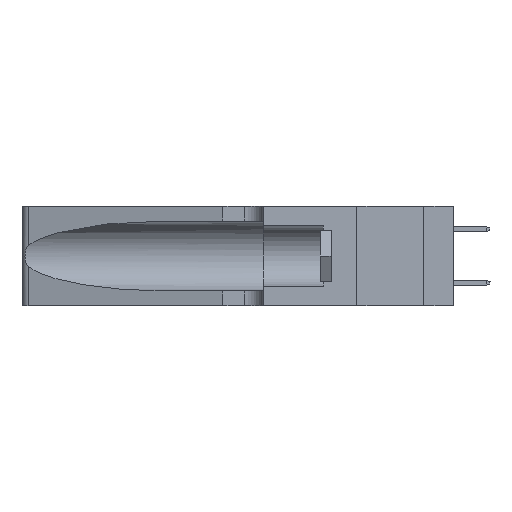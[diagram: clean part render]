
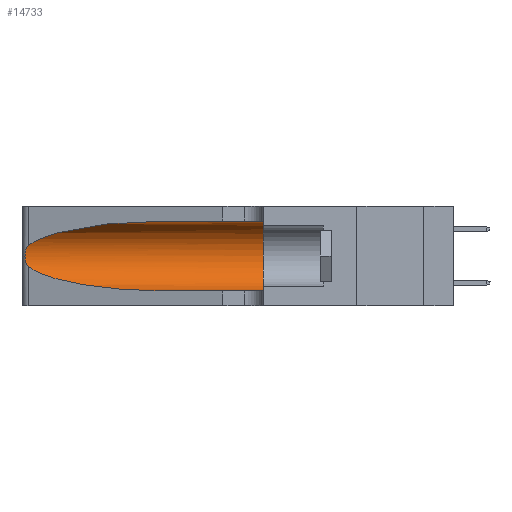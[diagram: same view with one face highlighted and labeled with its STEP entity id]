
A CAD part, left-side view. The second image highlights one B-rep face of the part: STEP entity #14733.
In plain terms, the highlighted cylindrical face has radius 3.308 mm (diameter 6.617 mm), a partial arc.
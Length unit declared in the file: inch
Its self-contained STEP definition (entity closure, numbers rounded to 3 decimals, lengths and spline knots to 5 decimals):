
#39 = CYLINDRICAL_SURFACE ( 'NONE', #864, 0.13025 ) ;
#864 = AXIS2_PLACEMENT_3D ( 'NONE', #15538, #2279, #7613 ) ;
#965 = ORIENTED_EDGE ( 'NONE', *, *, #1221, .F. ) ;
#1221 = EDGE_CURVE ( 'NONE', #31460, #3179, #30918, .T. ) ;
#1354 = CARTESIAN_POINT ( 'NONE',  ( 0.26075, 1.23896, 0.178 ) ) ;
#1527 = CARTESIAN_POINT ( 'NONE',  ( 0.26075, 1.23896, 0.19203 ) ) ;
#1654 = VERTEX_POINT ( 'NONE', #29854 ) ;
#1862 = VERTEX_POINT ( 'NONE', #2732 ) ;
#2131 = EDGE_CURVE ( 'NONE', #1654, #1862, #22072, .T. ) ;
#2279 = DIRECTION ( 'NONE',  ( 0., -1., 0. ) ) ;
#2346 = ORIENTED_EDGE ( 'NONE', *, *, #2131, .T. ) ;
#2530 = CARTESIAN_POINT ( 'NONE',  ( 0.1305, 0.72297, 0.31525 ) ) ;
#2732 = CARTESIAN_POINT ( 'NONE',  ( 0.25487, 1.22718, 0.14631 ) ) ;
#3179 = VERTEX_POINT ( 'NONE', #7120 ) ;
#5054 = CARTESIAN_POINT ( 'NONE',  ( 0.1305, 0.72297, 0.05475 ) ) ;
#5579 = AXIS2_PLACEMENT_3D ( 'NONE', #21646, #8551, #21817 ) ;
#6100 = ORIENTED_EDGE ( 'NONE', *, *, #20567, .F. ) ;
#6348 = CARTESIAN_POINT ( 'NONE',  ( 0.25487, 1.22718, 0.22369 ) ) ;
#6790 = LINE ( 'NONE', #27851, #25215 ) ;
#7036 = CARTESIAN_POINT ( 'NONE',  ( 0.25487, 1.22718, 0.14631 ) ) ;
#7120 = CARTESIAN_POINT ( 'NONE',  ( 0.1305, 0.35, 0.05475 ) ) ;
#7125 = CARTESIAN_POINT ( 'NONE',  ( 0.25487, 1.22718, 0.14631 ) ) ;
#7238 = CARTESIAN_POINT ( 'NONE',  ( 0.1305, 1.61858, 0.05475 ) ) ;
#7613 = DIRECTION ( 'NONE',  ( 0., 0., -1. ) ) ;
#8551 = DIRECTION ( 'NONE',  ( 0., 1., 0. ) ) ;
#9964 = CARTESIAN_POINT ( 'NONE',  ( 0.18966, 0.96281, 0.31525 ) ) ;
#10334 = LINE ( 'NONE', #7238, #25670 ) ;
#11707 = CARTESIAN_POINT ( 'NONE',  ( 0.25639, 1.23186, 0.15144 ) ) ;
#12054 = CARTESIAN_POINT ( 'NONE',  ( 0.25555, 1.22993, 0.14849 ) ) ;
#13056 = CARTESIAN_POINT ( 'NONE',  ( 0.25487, 1.22718, 0.22369 ) ) ;
#13820 = ORIENTED_EDGE ( 'NONE', *, *, #17818, .T. ) ;
#14646 = CARTESIAN_POINT ( 'NONE',  ( 0.1305, 0.35, 0.31525 ) ) ;
#14733 = ADVANCED_FACE ( 'NONE', ( #15710 ), #39, .F. ) ;
#15238 = EDGE_CURVE ( 'NONE', #31876, #3179, #10334, .T. ) ;
#15380 = CARTESIAN_POINT ( 'NONE',  ( 0.18966, 0.96281, 0.05475 ) ) ;
#15538 = CARTESIAN_POINT ( 'NONE',  ( 0.1305, 1.61858, 0.185 ) ) ;
#15710 = FACE_OUTER_BOUND ( 'NONE', #19893, .T. ) ;
#15809 = CARTESIAN_POINT ( 'NONE',  ( 0.2373, 1.15595, 0.28018 ) ) ;
#16860 = CARTESIAN_POINT ( 'NONE',  ( 0.25854, 1.2359, 0.20912 ) ) ;
#17818 = EDGE_CURVE ( 'NONE', #1862, #31876, #25485, .T. ) ;
#19546 =( BOUNDED_CURVE ( )  B_SPLINE_CURVE ( 3, ( #2530, #9964, #15809, #13056 ),
 .UNSPECIFIED., .F., .F. ) 
 B_SPLINE_CURVE_WITH_KNOTS ( ( 4, 4 ),
 ( 1.5708, 2.84003 ),
 .UNSPECIFIED. ) 
 CURVE ( )  GEOMETRIC_REPRESENTATION_ITEM ( )  RATIONAL_B_SPLINE_CURVE ( ( 1., 0.87, 0.87, 1. ) ) 
 REPRESENTATION_ITEM ( '' )  );
#19893 = EDGE_LOOP ( 'NONE', ( #32483, #2346, #13820, #28740, #965, #6100 ) ) ;
#20567 = EDGE_CURVE ( 'NONE', #24941, #31460, #6790, .T. ) ;
#21646 = CARTESIAN_POINT ( 'NONE',  ( 0.1305, 0.35, 0.185 ) ) ;
#21817 = DIRECTION ( 'NONE',  ( 0., 0., 1. ) ) ;
#22072 = B_SPLINE_CURVE_WITH_KNOTS ( 'NONE', 3,
 ( #6348, #24802, #22586, #30490, #16860, #27404, #1527, #1354, #30156, #27752, #25148, #11707, #12054, #7036 ),
 .UNSPECIFIED., .F., .F.,
 ( 4, 2, 2, 2, 2, 2, 4 ),
 ( 0., 0.00027, 0.00053, 0.00107, 0.0016, 0.00187, 0.00214 ),
 .UNSPECIFIED. ) ;
#22586 = CARTESIAN_POINT ( 'NONE',  ( 0.25639, 1.23184, 0.21858 ) ) ;
#22842 = CARTESIAN_POINT ( 'NONE',  ( 0.2373, 1.15595, 0.08982 ) ) ;
#23287 = DIRECTION ( 'NONE',  ( 0., -1., 0. ) ) ;
#24802 = CARTESIAN_POINT ( 'NONE',  ( 0.25555, 1.22994, 0.2215 ) ) ;
#24941 = VERTEX_POINT ( 'NONE', #30001 ) ;
#25148 = CARTESIAN_POINT ( 'NONE',  ( 0.25789, 1.23486, 0.15765 ) ) ;
#25215 = VECTOR ( 'NONE', #30588, 39.37008 ) ;
#25485 =( BOUNDED_CURVE ( )  B_SPLINE_CURVE ( 3, ( #7125, #22842, #15380, #5054 ),
 .UNSPECIFIED., .F., .F. ) 
 B_SPLINE_CURVE_WITH_KNOTS ( ( 4, 4 ),
 ( 3.44316, 4.71239 ),
 .UNSPECIFIED. ) 
 CURVE ( )  GEOMETRIC_REPRESENTATION_ITEM ( )  RATIONAL_B_SPLINE_CURVE ( ( 1., 0.87, 0.87, 1. ) ) 
 REPRESENTATION_ITEM ( '' )  );
#25670 = VECTOR ( 'NONE', #23287, 39.37008 ) ;
#27266 = EDGE_CURVE ( 'NONE', #24941, #1654, #19546, .T. ) ;
#27404 = CARTESIAN_POINT ( 'NONE',  ( 0.26018, 1.23835, 0.19895 ) ) ;
#27752 = CARTESIAN_POINT ( 'NONE',  ( 0.25856, 1.23593, 0.16098 ) ) ;
#27851 = CARTESIAN_POINT ( 'NONE',  ( 0.1305, 1.61858, 0.31525 ) ) ;
#28740 = ORIENTED_EDGE ( 'NONE', *, *, #15238, .T. ) ;
#29854 = CARTESIAN_POINT ( 'NONE',  ( 0.25487, 1.22718, 0.22369 ) ) ;
#30001 = CARTESIAN_POINT ( 'NONE',  ( 0.1305, 0.72297, 0.31525 ) ) ;
#30133 = CARTESIAN_POINT ( 'NONE',  ( 0.1305, 0.72297, 0.05475 ) ) ;
#30156 = CARTESIAN_POINT ( 'NONE',  ( 0.26017, 1.23833, 0.17102 ) ) ;
#30490 = CARTESIAN_POINT ( 'NONE',  ( 0.25787, 1.23484, 0.2124 ) ) ;
#30588 = DIRECTION ( 'NONE',  ( 0., -1., 0. ) ) ;
#30918 = CIRCLE ( 'NONE', #5579, 0.13025 ) ;
#31460 = VERTEX_POINT ( 'NONE', #14646 ) ;
#31876 = VERTEX_POINT ( 'NONE', #30133 ) ;
#32483 = ORIENTED_EDGE ( 'NONE', *, *, #27266, .T. ) ;
